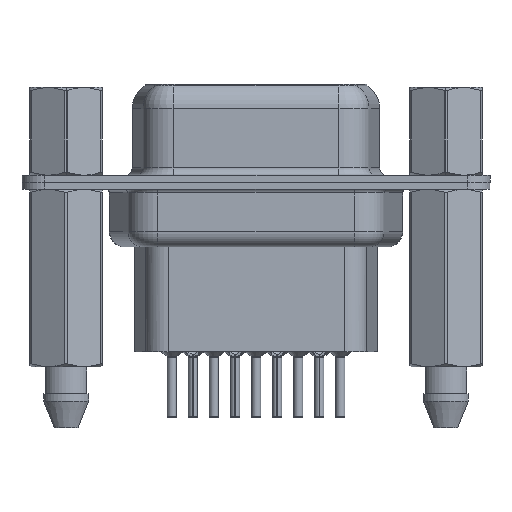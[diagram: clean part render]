
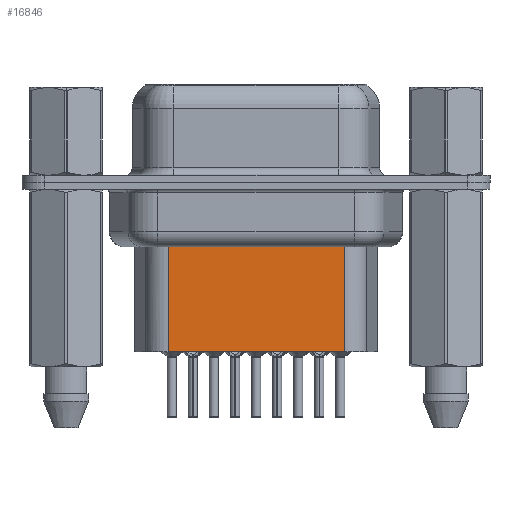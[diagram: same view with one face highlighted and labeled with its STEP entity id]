
A CAD part, front view. The second image highlights one B-rep face of the part: STEP entity #16846.
In plain terms, the highlighted planar face has unit normal (0, -1, 0).
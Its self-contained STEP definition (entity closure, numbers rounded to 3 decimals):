
#691 = EDGE_CURVE ( 'NONE', #17894, #24749, #8089, .T. ) ;
#2734 = CARTESIAN_POINT ( 'NONE',  ( 6.706, -3.5, -11.15 ) ) ;
#2872 = LINE ( 'NONE', #24330, #11912 ) ;
#2954 = DIRECTION ( 'NONE',  ( 1., 0., 0. ) ) ;
#3501 = DIRECTION ( 'NONE',  ( 0., 0., -1. ) ) ;
#4892 = PLANE ( 'NONE',  #19682 ) ;
#5501 = LINE ( 'NONE', #2734, #5666 ) ;
#5666 = VECTOR ( 'NONE', #27111, 1000. ) ;
#7606 = ORIENTED_EDGE ( 'NONE', *, *, #9502, .F. ) ;
#8089 = LINE ( 'NONE', #20362, #11974 ) ;
#8759 = CARTESIAN_POINT ( 'NONE',  ( 6.706, -3.5, -11.15 ) ) ;
#9500 = EDGE_CURVE ( 'NONE', #17894, #19079, #2872, .T. ) ;
#9502 = EDGE_CURVE ( 'NONE', #24749, #15971, #5501, .T. ) ;
#11665 = LINE ( 'NONE', #15694, #22360 ) ;
#11912 = VECTOR ( 'NONE', #20273, 1000. ) ;
#11974 = VECTOR ( 'NONE', #3501, 1000. ) ;
#13048 = ORIENTED_EDGE ( 'NONE', *, *, #22289, .T. ) ;
#15694 = CARTESIAN_POINT ( 'NONE',  ( 6.706, -3.5, -3.1 ) ) ;
#15971 = VERTEX_POINT ( 'NONE', #8759 ) ;
#16846 = ADVANCED_FACE ( 'NONE', ( #22047 ), #4892, .T. ) ;
#17894 = VERTEX_POINT ( 'NONE', #19724 ) ;
#18709 = CARTESIAN_POINT ( 'NONE',  ( 6.706, -3.5, -4.097 ) ) ;
#19079 = VERTEX_POINT ( 'NONE', #18709 ) ;
#19682 = AXIS2_PLACEMENT_3D ( 'NONE', #24133, #22177, #2954 ) ;
#19724 = CARTESIAN_POINT ( 'NONE',  ( 18.294, -3.5, -4.097 ) ) ;
#20273 = DIRECTION ( 'NONE',  ( -1., 0., 0. ) ) ;
#20362 = CARTESIAN_POINT ( 'NONE',  ( 18.294, -3.5, -3.1 ) ) ;
#20441 = ORIENTED_EDGE ( 'NONE', *, *, #691, .F. ) ;
#21323 = CARTESIAN_POINT ( 'NONE',  ( 18.294, -3.5, -11.15 ) ) ;
#21905 = ORIENTED_EDGE ( 'NONE', *, *, #9500, .T. ) ;
#22047 = FACE_OUTER_BOUND ( 'NONE', #27558, .T. ) ;
#22096 = DIRECTION ( 'NONE',  ( 0., 0., -1. ) ) ;
#22177 = DIRECTION ( 'NONE',  ( 0., -1., 0. ) ) ;
#22289 = EDGE_CURVE ( 'NONE', #19079, #15971, #11665, .T. ) ;
#22360 = VECTOR ( 'NONE', #22096, 1000. ) ;
#24133 = CARTESIAN_POINT ( 'NONE',  ( 6.706, -3.5, -3.1 ) ) ;
#24330 = CARTESIAN_POINT ( 'NONE',  ( 6.459, -3.5, -4.097 ) ) ;
#24749 = VERTEX_POINT ( 'NONE', #21323 ) ;
#27111 = DIRECTION ( 'NONE',  ( -1., 0., 0. ) ) ;
#27558 = EDGE_LOOP ( 'NONE', ( #20441, #21905, #13048, #7606 ) ) ;
